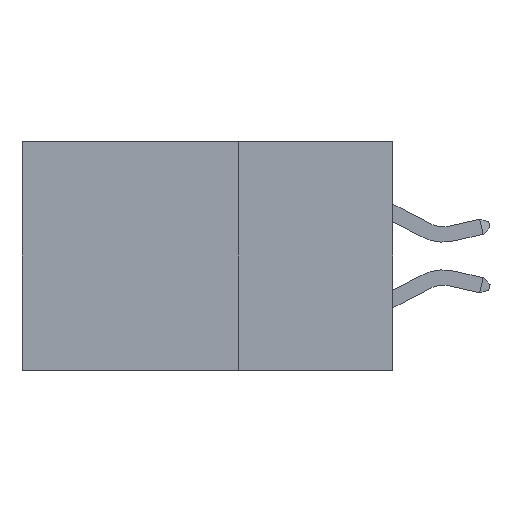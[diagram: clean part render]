
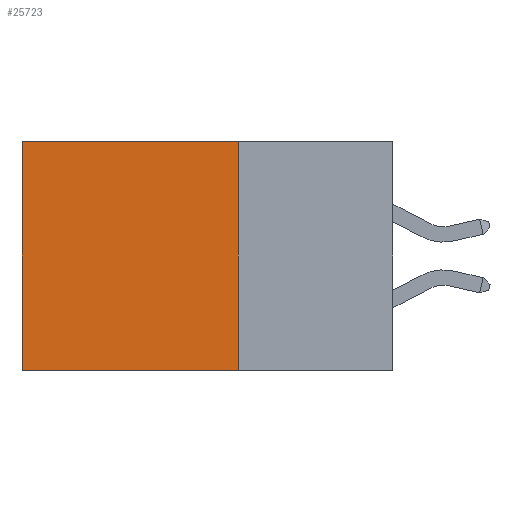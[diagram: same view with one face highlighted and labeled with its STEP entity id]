
A CAD part, left-side view. The second image highlights one B-rep face of the part: STEP entity #25723.
In plain terms, the highlighted planar face has unit normal (-1, 0, 0).
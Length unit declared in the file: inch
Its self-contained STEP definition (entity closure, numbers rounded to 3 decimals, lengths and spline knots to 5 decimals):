
#369 = CARTESIAN_POINT ( 'NONE',  ( 0.2875, 0.25, -0.37 ) ) ;
#1439 = CARTESIAN_POINT ( 'NONE',  ( 0.2875, 0.25, 0. ) ) ;
#1531 = DIRECTION ( 'NONE',  ( 0., 1., 0. ) ) ;
#2712 = ORIENTED_EDGE ( 'NONE', *, *, #21991, .F. ) ;
#2888 = LINE ( 'NONE', #8906, #16340 ) ;
#3253 = VERTEX_POINT ( 'NONE', #7306 ) ;
#4810 = CARTESIAN_POINT ( 'NONE',  ( 0.2875, 0.25, 0. ) ) ;
#5630 = LINE ( 'NONE', #25663, #15281 ) ;
#6962 = LINE ( 'NONE', #1439, #20413 ) ;
#7306 = CARTESIAN_POINT ( 'NONE',  ( 0.2875, 0.25, 0. ) ) ;
#8714 = DIRECTION ( 'NONE',  ( 0., 0., -1. ) ) ;
#8906 = CARTESIAN_POINT ( 'NONE',  ( 0.2875, 0.25, 0. ) ) ;
#9152 = PLANE ( 'NONE',  #19606 ) ;
#9367 = VERTEX_POINT ( 'NONE', #16809 ) ;
#10219 = VECTOR ( 'NONE', #23938, 39.37008 ) ;
#10934 = EDGE_LOOP ( 'NONE', ( #28221, #20533, #2712, #22588 ) ) ;
#12617 = LINE ( 'NONE', #13228, #10219 ) ;
#12868 = CARTESIAN_POINT ( 'NONE',  ( 0.2875, 0.6, 0. ) ) ;
#13228 = CARTESIAN_POINT ( 'NONE',  ( 0.2875, 0.6, 0. ) ) ;
#14623 = EDGE_CURVE ( 'NONE', #28576, #9367, #5630, .T. ) ;
#15278 = EDGE_CURVE ( 'NONE', #3253, #19963, #6962, .T. ) ;
#15281 = VECTOR ( 'NONE', #25472, 39.37008 ) ;
#15896 = DIRECTION ( 'NONE',  ( 1., 0., 0. ) ) ;
#16340 = VECTOR ( 'NONE', #8714, 39.37008 ) ;
#16809 = CARTESIAN_POINT ( 'NONE',  ( 0.2875, 0.6, -0.37 ) ) ;
#19606 = AXIS2_PLACEMENT_3D ( 'NONE', #4810, #15896, #20526 ) ;
#19963 = VERTEX_POINT ( 'NONE', #12868 ) ;
#20413 = VECTOR ( 'NONE', #1531, 39.37008 ) ;
#20526 = DIRECTION ( 'NONE',  ( 0., 0., -1. ) ) ;
#20533 = ORIENTED_EDGE ( 'NONE', *, *, #14623, .F. ) ;
#20675 = EDGE_CURVE ( 'NONE', #19963, #9367, #12617, .T. ) ;
#21991 = EDGE_CURVE ( 'NONE', #3253, #28576, #2888, .T. ) ;
#22588 = ORIENTED_EDGE ( 'NONE', *, *, #15278, .T. ) ;
#23938 = DIRECTION ( 'NONE',  ( 0., 0., -1. ) ) ;
#25472 = DIRECTION ( 'NONE',  ( 0., 1., 0. ) ) ;
#25663 = CARTESIAN_POINT ( 'NONE',  ( 0.2875, 0.25, -0.37 ) ) ;
#25723 = ADVANCED_FACE ( 'NONE', ( #28456 ), #9152, .F. ) ;
#28221 = ORIENTED_EDGE ( 'NONE', *, *, #20675, .T. ) ;
#28456 = FACE_OUTER_BOUND ( 'NONE', #10934, .T. ) ;
#28576 = VERTEX_POINT ( 'NONE', #369 ) ;
